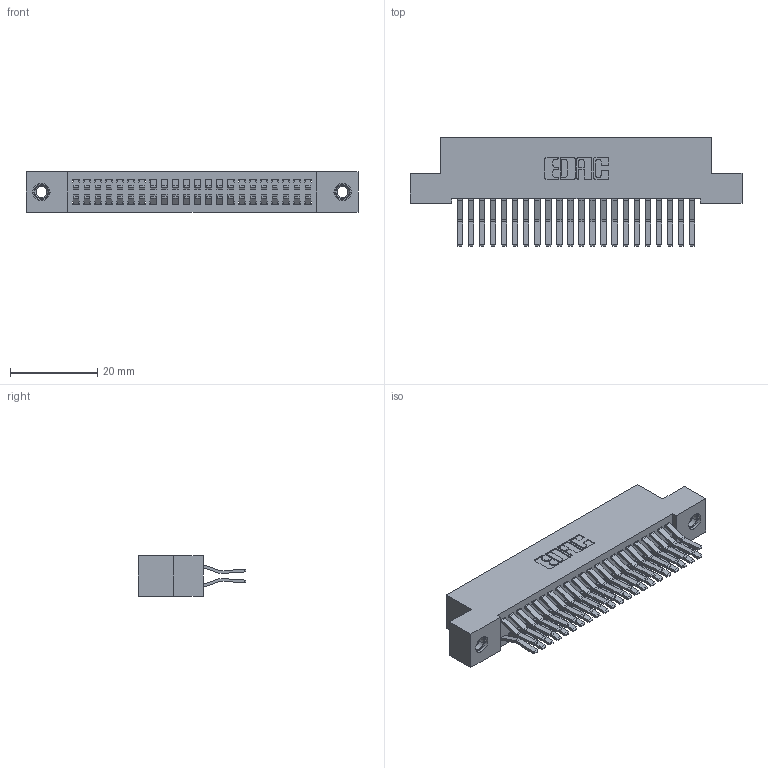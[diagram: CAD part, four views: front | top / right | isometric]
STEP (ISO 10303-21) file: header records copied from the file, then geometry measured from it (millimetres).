
FILE_DESCRIPTION (( 'STEP AP203' ), '1' );
FILE_NAME ('392-044-560-207.STEP', '2019-10-07T22:49:41', ( '' ), ( '' ), 'SwSTEP 2.0', 'SolidWorks 2016', '' );
FILE_SCHEMA (( 'CONFIG_CONTROL_DESIGN' ));
Length unit declared in the file: inch
Products named in the file (4): 345-292-001_560 Tail; 345-250-001_345-250-005-103; 392-044-560-207; 342 Part_TI
Assembly tree (47 placements, depth 2):
  392-044-560-207
    342 Part_TI
    345-292-001_560 Tail  x44
    345-250-001_345-250-005-103  x2
Bounding box: 76.2 x 24.78 x 9.4 mm (x, y, z)
Volume: 7028.1 mm3; surface area: 11665.6 mm2
Topology: 47 solids, 47 shells, 2546 faces, 7519 edges, 4946 vertices
Faces by surface type: plane 1682, cylinder 848, cone 12, torus 4
Entity records: 17882 total; most frequent: CARTESIAN_POINT 2969, ORIENTED_EDGE 2898, DIRECTION 2607, EDGE_CURVE 1449, LINE 1297, VECTOR 1297, VERTEX_POINT 960, AXIS2_PLACEMENT_3D 655
